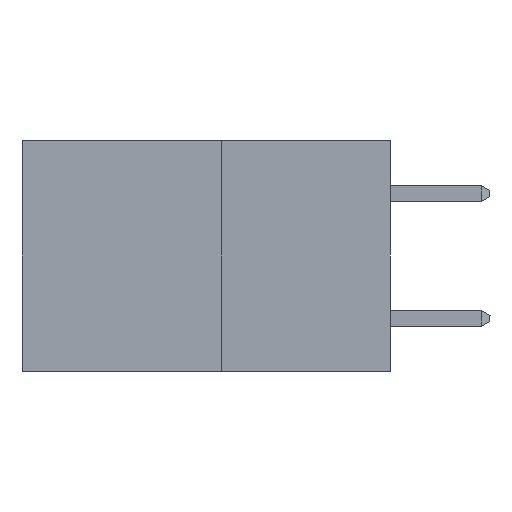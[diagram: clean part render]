
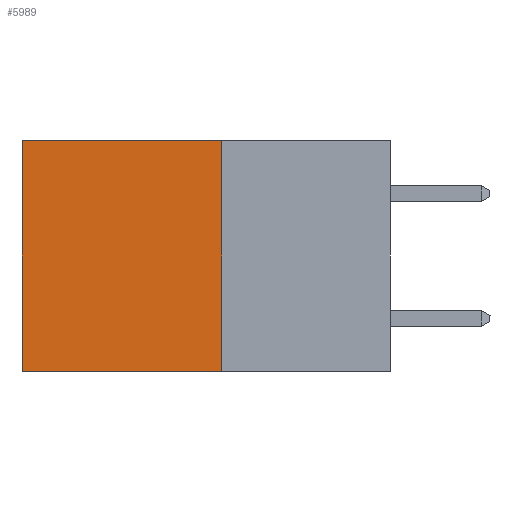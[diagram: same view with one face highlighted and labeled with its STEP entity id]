
A CAD part, left-side view. The second image highlights one B-rep face of the part: STEP entity #5989.
In plain terms, the highlighted planar face has unit normal (-1, 0, 0).
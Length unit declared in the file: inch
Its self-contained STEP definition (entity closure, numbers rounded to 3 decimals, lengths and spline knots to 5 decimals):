
#240 = VERTEX_POINT ( 'NONE', #5732 ) ;
#796 = FACE_OUTER_BOUND ( 'NONE', #854, .T. ) ;
#854 = EDGE_LOOP ( 'NONE', ( #6297, #866, #7146, #1878 ) ) ;
#866 = ORIENTED_EDGE ( 'NONE', *, *, #7088, .F. ) ;
#1507 = VERTEX_POINT ( 'NONE', #7164 ) ;
#1878 = ORIENTED_EDGE ( 'NONE', *, *, #5920, .T. ) ;
#2190 = LINE ( 'NONE', #8508, #6019 ) ;
#2216 = VECTOR ( 'NONE', #5861, 39.37008 ) ;
#2453 = LINE ( 'NONE', #6072, #2216 ) ;
#4043 = AXIS2_PLACEMENT_3D ( 'NONE', #4752, #4726, #4704 ) ;
#4526 = VECTOR ( 'NONE', #5500, 39.37008 ) ;
#4704 = DIRECTION ( 'NONE',  ( 0., 0., -1. ) ) ;
#4726 = DIRECTION ( 'NONE',  ( 1., 0., 0. ) ) ;
#4752 = CARTESIAN_POINT ( 'NONE',  ( 0.277, 0.27, -0.37 ) ) ;
#4767 = PLANE ( 'NONE',  #4043 ) ;
#5096 = VERTEX_POINT ( 'NONE', #7951 ) ;
#5500 = DIRECTION ( 'NONE',  ( 0., 0., -1. ) ) ;
#5675 = DIRECTION ( 'NONE',  ( 0., 1., 0. ) ) ;
#5732 = CARTESIAN_POINT ( 'NONE',  ( 0.277, 0.59, -0.37 ) ) ;
#5861 = DIRECTION ( 'NONE',  ( 0., 1., 0. ) ) ;
#5886 = CARTESIAN_POINT ( 'NONE',  ( 0.277, 0.27, 0. ) ) ;
#5920 = EDGE_CURVE ( 'NONE', #7036, #5096, #6137, .T. ) ;
#5989 = ADVANCED_FACE ( 'NONE', ( #796 ), #4767, .F. ) ;
#6019 = VECTOR ( 'NONE', #7138, 39.37008 ) ;
#6072 = CARTESIAN_POINT ( 'NONE',  ( 0.277, 0.27, -0.37 ) ) ;
#6137 = LINE ( 'NONE', #5886, #7500 ) ;
#6297 = ORIENTED_EDGE ( 'NONE', *, *, #8811, .T. ) ;
#6959 = CARTESIAN_POINT ( 'NONE',  ( 0.277, 0.27, 0. ) ) ;
#7036 = VERTEX_POINT ( 'NONE', #6959 ) ;
#7088 = EDGE_CURVE ( 'NONE', #1507, #240, #2453, .T. ) ;
#7138 = DIRECTION ( 'NONE',  ( 0., 0., -1. ) ) ;
#7146 = ORIENTED_EDGE ( 'NONE', *, *, #8433, .F. ) ;
#7164 = CARTESIAN_POINT ( 'NONE',  ( 0.277, 0.27, -0.37 ) ) ;
#7500 = VECTOR ( 'NONE', #5675, 39.37008 ) ;
#7951 = CARTESIAN_POINT ( 'NONE',  ( 0.277, 0.59, 0. ) ) ;
#8268 = CARTESIAN_POINT ( 'NONE',  ( 0.277, 0.59, -0.37 ) ) ;
#8433 = EDGE_CURVE ( 'NONE', #7036, #1507, #2190, .T. ) ;
#8508 = CARTESIAN_POINT ( 'NONE',  ( 0.277, 0.27, -0.37 ) ) ;
#8666 = LINE ( 'NONE', #8268, #4526 ) ;
#8811 = EDGE_CURVE ( 'NONE', #5096, #240, #8666, .T. ) ;
